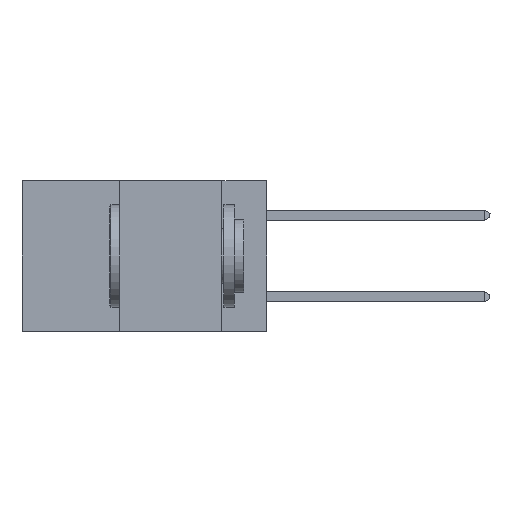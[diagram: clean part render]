
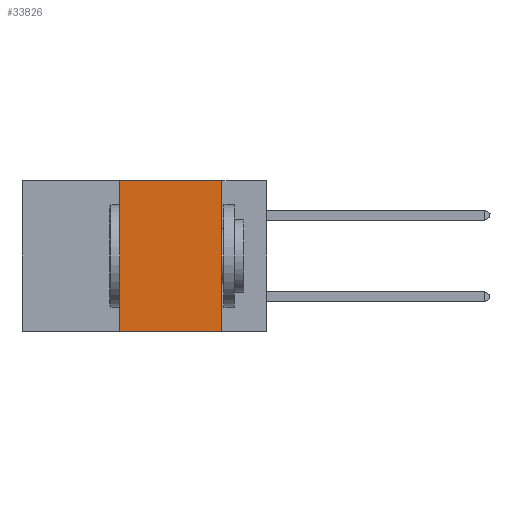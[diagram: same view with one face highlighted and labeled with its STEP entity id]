
A CAD part, left-side view. The second image highlights one B-rep face of the part: STEP entity #33826.
In plain terms, the highlighted planar face has unit normal (-1, 0, 0).
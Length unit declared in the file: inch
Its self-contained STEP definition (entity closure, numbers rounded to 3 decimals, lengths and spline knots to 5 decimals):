
#67 = CARTESIAN_POINT ( 'NONE',  ( 0., 0.11, 0. ) ) ;
#778 = DIRECTION ( 'NONE',  ( 0., 0., -1. ) ) ;
#3093 = CARTESIAN_POINT ( 'NONE',  ( 0., 0.36, 0. ) ) ;
#4715 = FACE_OUTER_BOUND ( 'NONE', #17569, .T. ) ;
#6773 = LINE ( 'NONE', #3093, #37972 ) ;
#9718 = VECTOR ( 'NONE', #31392, 39.37008 ) ;
#10317 = VERTEX_POINT ( 'NONE', #25787 ) ;
#10570 = DIRECTION ( 'NONE',  ( 0., 0., 1. ) ) ;
#13663 = DIRECTION ( 'NONE',  ( 0., -1., 0. ) ) ;
#13900 = VECTOR ( 'NONE', #29934, 39.37008 ) ;
#15653 = VERTEX_POINT ( 'NONE', #28453 ) ;
#15737 = VERTEX_POINT ( 'NONE', #32052 ) ;
#16283 = VERTEX_POINT ( 'NONE', #67 ) ;
#17569 = EDGE_LOOP ( 'NONE', ( #35886, #33186, #18644, #30618 ) ) ;
#18644 = ORIENTED_EDGE ( 'NONE', *, *, #36302, .F. ) ;
#19460 = LINE ( 'NONE', #26362, #13900 ) ;
#25490 = VECTOR ( 'NONE', #13663, 39.37008 ) ;
#25787 = CARTESIAN_POINT ( 'NONE',  ( 0., 0.36, 0. ) ) ;
#26362 = CARTESIAN_POINT ( 'NONE',  ( 0., 0.6, 0. ) ) ;
#27827 = AXIS2_PLACEMENT_3D ( 'NONE', #42981, #28967, #778 ) ;
#28096 = CARTESIAN_POINT ( 'NONE',  ( 0., 0.11, 0. ) ) ;
#28453 = CARTESIAN_POINT ( 'NONE',  ( 0., 0.36, -0.37 ) ) ;
#28967 = DIRECTION ( 'NONE',  ( 1., 0., 0. ) ) ;
#29131 = PLANE ( 'NONE',  #27827 ) ;
#29934 = DIRECTION ( 'NONE',  ( 0., -1., 0. ) ) ;
#30618 = ORIENTED_EDGE ( 'NONE', *, *, #44975, .T. ) ;
#31392 = DIRECTION ( 'NONE',  ( 0., 0., -1. ) ) ;
#32052 = CARTESIAN_POINT ( 'NONE',  ( 0., 0.11, -0.37 ) ) ;
#32707 = LINE ( 'NONE', #41792, #25490 ) ;
#33186 = ORIENTED_EDGE ( 'NONE', *, *, #37415, .F. ) ;
#33826 = ADVANCED_FACE ( 'NONE', ( #4715 ), #29131, .F. ) ;
#34959 = EDGE_CURVE ( 'NONE', #16283, #15737, #36433, .T. ) ;
#35886 = ORIENTED_EDGE ( 'NONE', *, *, #34959, .F. ) ;
#36302 = EDGE_CURVE ( 'NONE', #15653, #10317, #6773, .T. ) ;
#36433 = LINE ( 'NONE', #28096, #9718 ) ;
#37415 = EDGE_CURVE ( 'NONE', #10317, #16283, #19460, .T. ) ;
#37972 = VECTOR ( 'NONE', #10570, 39.37008 ) ;
#41792 = CARTESIAN_POINT ( 'NONE',  ( 0., 0.6, -0.37 ) ) ;
#42981 = CARTESIAN_POINT ( 'NONE',  ( 0., 0.6, 0. ) ) ;
#44975 = EDGE_CURVE ( 'NONE', #15653, #15737, #32707, .T. ) ;
